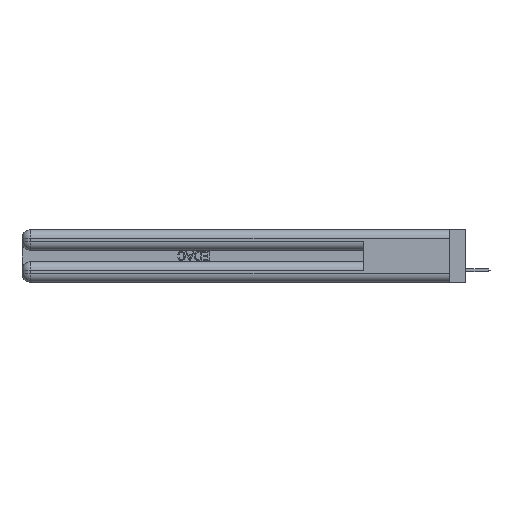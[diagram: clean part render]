
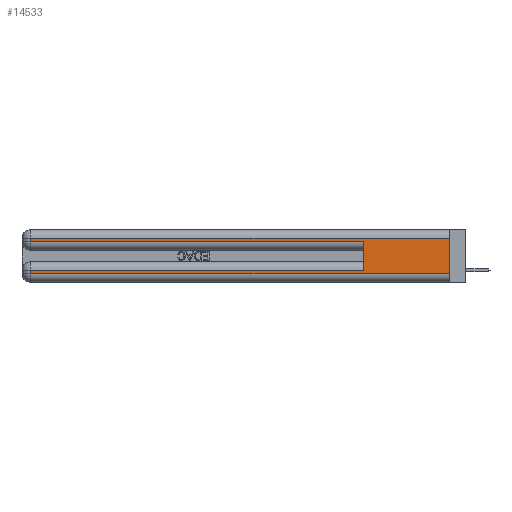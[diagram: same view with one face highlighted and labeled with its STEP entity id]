
A CAD part, left-side view. The second image highlights one B-rep face of the part: STEP entity #14533.
In plain terms, the highlighted planar face has unit normal (-1, 0, 0).
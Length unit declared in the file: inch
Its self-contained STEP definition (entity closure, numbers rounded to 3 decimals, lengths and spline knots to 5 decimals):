
#539 = ORIENTED_EDGE ( 'NONE', *, *, #14309, .T. ) ;
#1235 = EDGE_CURVE ( 'NONE', #11497, #3669, #19350, .T. ) ;
#1980 = LINE ( 'NONE', #3914, #14510 ) ;
#2230 = ORIENTED_EDGE ( 'NONE', *, *, #10667, .T. ) ;
#2241 = DIRECTION ( 'NONE',  ( 0., -1., 0. ) ) ;
#2426 = ORIENTED_EDGE ( 'NONE', *, *, #22146, .T. ) ;
#2966 = DIRECTION ( 'NONE',  ( 1., 0., 0. ) ) ;
#3669 = VERTEX_POINT ( 'NONE', #12446 ) ;
#3914 = CARTESIAN_POINT ( 'NONE',  ( 0., 0., 0.085 ) ) ;
#4203 = ORIENTED_EDGE ( 'NONE', *, *, #19374, .F. ) ;
#4270 = LINE ( 'NONE', #29257, #32894 ) ;
#4973 = DIRECTION ( 'NONE',  ( 0., 0., -1. ) ) ;
#5215 = CARTESIAN_POINT ( 'NONE',  ( 0., 2.94, 0.37 ) ) ;
#5893 = DIRECTION ( 'NONE',  ( 0., 0., -1. ) ) ;
#6203 = VECTOR ( 'NONE', #2241, 39.37008 ) ;
#6769 = CARTESIAN_POINT ( 'NONE',  ( 0., 2.94, 0.085 ) ) ;
#6839 = ORIENTED_EDGE ( 'NONE', *, *, #29032, .T. ) ;
#10000 = CARTESIAN_POINT ( 'NONE',  ( 0., 0.6, 0.285 ) ) ;
#10035 = FACE_OUTER_BOUND ( 'NONE', #23686, .T. ) ;
#10667 = EDGE_CURVE ( 'NONE', #34256, #13397, #34708, .T. ) ;
#11497 = VERTEX_POINT ( 'NONE', #6769 ) ;
#11908 = DIRECTION ( 'NONE',  ( 0., -1., 0. ) ) ;
#12446 = CARTESIAN_POINT ( 'NONE',  ( 0., 2.94, 0.06 ) ) ;
#12488 = EDGE_CURVE ( 'NONE', #3669, #20103, #13586, .T. ) ;
#13145 = VECTOR ( 'NONE', #11908, 39.37008 ) ;
#13254 = CARTESIAN_POINT ( 'NONE',  ( 0., 0., 0.37 ) ) ;
#13397 = VERTEX_POINT ( 'NONE', #35434 ) ;
#13586 = LINE ( 'NONE', #31992, #13145 ) ;
#13598 = ORIENTED_EDGE ( 'NONE', *, *, #13873, .F. ) ;
#13873 = EDGE_CURVE ( 'NONE', #34256, #20103, #18902, .T. ) ;
#14309 = EDGE_CURVE ( 'NONE', #35547, #11497, #1980, .T. ) ;
#14510 = VECTOR ( 'NONE', #32801, 39.37008 ) ;
#14533 = ADVANCED_FACE ( 'NONE', ( #10035 ), #25677, .F. ) ;
#16949 = LINE ( 'NONE', #21944, #6203 ) ;
#17765 = VECTOR ( 'NONE', #31831, 39.37008 ) ;
#18902 = LINE ( 'NONE', #13254, #27400 ) ;
#19350 = LINE ( 'NONE', #5215, #33612 ) ;
#19367 = CARTESIAN_POINT ( 'NONE',  ( 0., 2.94, 0.285 ) ) ;
#19374 = EDGE_CURVE ( 'NONE', #35547, #32763, #4270, .T. ) ;
#20099 = ORIENTED_EDGE ( 'NONE', *, *, #1235, .T. ) ;
#20103 = VERTEX_POINT ( 'NONE', #20935 ) ;
#20377 = CARTESIAN_POINT ( 'NONE',  ( 0., 0.6, 0.085 ) ) ;
#20544 = DIRECTION ( 'NONE',  ( 0., 0., 1. ) ) ;
#20900 = CARTESIAN_POINT ( 'NONE',  ( 0., 0., 0.31 ) ) ;
#20935 = CARTESIAN_POINT ( 'NONE',  ( 0., 0., 0.06 ) ) ;
#21915 = DIRECTION ( 'NONE',  ( 0., 0., -1. ) ) ;
#21944 = CARTESIAN_POINT ( 'NONE',  ( 0., 0., 0.285 ) ) ;
#22146 = EDGE_CURVE ( 'NONE', #30926, #32763, #16949, .T. ) ;
#23686 = EDGE_LOOP ( 'NONE', ( #13598, #2230, #6839, #2426, #4203, #539, #20099, #36819 ) ) ;
#24881 = DIRECTION ( 'NONE',  ( 0., 0., -1. ) ) ;
#25431 = CARTESIAN_POINT ( 'NONE',  ( 0., 0., 0.37 ) ) ;
#25677 = PLANE ( 'NONE',  #36499 ) ;
#25698 = VECTOR ( 'NONE', #21915, 39.37008 ) ;
#27400 = VECTOR ( 'NONE', #4973, 39.37008 ) ;
#28330 = CARTESIAN_POINT ( 'NONE',  ( 0., 0., 0.31 ) ) ;
#29032 = EDGE_CURVE ( 'NONE', #13397, #30926, #29661, .T. ) ;
#29257 = CARTESIAN_POINT ( 'NONE',  ( 0., 0.6, 0.145 ) ) ;
#29661 = LINE ( 'NONE', #33247, #25698 ) ;
#30926 = VERTEX_POINT ( 'NONE', #19367 ) ;
#31831 = DIRECTION ( 'NONE',  ( 0., 1., 0. ) ) ;
#31992 = CARTESIAN_POINT ( 'NONE',  ( 0., 0., 0.06 ) ) ;
#32763 = VERTEX_POINT ( 'NONE', #10000 ) ;
#32801 = DIRECTION ( 'NONE',  ( 0., 1., 0. ) ) ;
#32894 = VECTOR ( 'NONE', #20544, 39.37008 ) ;
#33247 = CARTESIAN_POINT ( 'NONE',  ( 0., 2.94, 0.37 ) ) ;
#33612 = VECTOR ( 'NONE', #24881, 39.37008 ) ;
#34256 = VERTEX_POINT ( 'NONE', #28330 ) ;
#34708 = LINE ( 'NONE', #20900, #17765 ) ;
#35434 = CARTESIAN_POINT ( 'NONE',  ( 0., 2.94, 0.31 ) ) ;
#35547 = VERTEX_POINT ( 'NONE', #20377 ) ;
#36499 = AXIS2_PLACEMENT_3D ( 'NONE', #25431, #2966, #5893 ) ;
#36819 = ORIENTED_EDGE ( 'NONE', *, *, #12488, .T. ) ;
